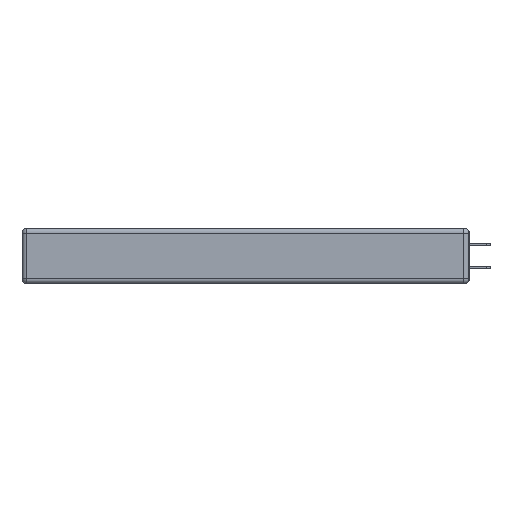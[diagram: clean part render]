
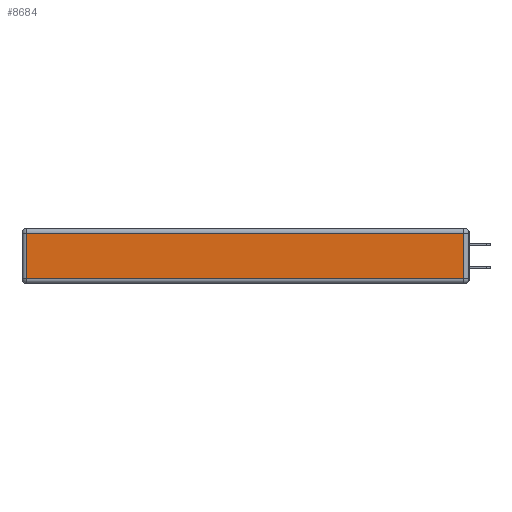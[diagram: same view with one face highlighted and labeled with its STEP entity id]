
A CAD part, left-side view. The second image highlights one B-rep face of the part: STEP entity #8684.
In plain terms, the highlighted planar face has unit normal (-1, 0, 0).
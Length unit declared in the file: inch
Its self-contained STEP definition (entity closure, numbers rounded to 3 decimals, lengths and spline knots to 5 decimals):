
#190 = LINE ( 'NONE', #18032, #3836 ) ;
#282 = DIRECTION ( 'NONE',  ( 0., 1., 0. ) ) ;
#2581 = VERTEX_POINT ( 'NONE', #12577 ) ;
#2840 = ORIENTED_EDGE ( 'NONE', *, *, #27368, .T. ) ;
#3521 = CARTESIAN_POINT ( 'NONE',  ( 0., 2.72, -0.313 ) ) ;
#3836 = VECTOR ( 'NONE', #12728, 39.37008 ) ;
#5255 = CARTESIAN_POINT ( 'NONE',  ( 0., 0.03, -0.313 ) ) ;
#5949 = VERTEX_POINT ( 'NONE', #33592 ) ;
#7208 = AXIS2_PLACEMENT_3D ( 'NONE', #22258, #24568, #11849 ) ;
#7485 = FACE_OUTER_BOUND ( 'NONE', #22815, .T. ) ;
#8135 = CARTESIAN_POINT ( 'NONE',  ( 0., 2.75, -0.03 ) ) ;
#8597 = CARTESIAN_POINT ( 'NONE',  ( 0., 2.72, -0.343 ) ) ;
#8684 = ADVANCED_FACE ( 'NONE', ( #7485 ), #8914, .T. ) ;
#8914 = PLANE ( 'NONE',  #7208 ) ;
#10251 = EDGE_CURVE ( 'NONE', #2581, #5949, #10608, .T. ) ;
#10278 = VECTOR ( 'NONE', #11177, 39.37008 ) ;
#10608 = LINE ( 'NONE', #8135, #11804 ) ;
#11177 = DIRECTION ( 'NONE',  ( 0., 0., -1. ) ) ;
#11804 = VECTOR ( 'NONE', #282, 39.37008 ) ;
#11849 = DIRECTION ( 'NONE',  ( 0., 0., 1. ) ) ;
#12577 = CARTESIAN_POINT ( 'NONE',  ( 0., 0.03, -0.03 ) ) ;
#12728 = DIRECTION ( 'NONE',  ( 0., -1., 0. ) ) ;
#15113 = ORIENTED_EDGE ( 'NONE', *, *, #27720, .T. ) ;
#15547 = VECTOR ( 'NONE', #23289, 39.37008 ) ;
#18032 = CARTESIAN_POINT ( 'NONE',  ( 0., 0., -0.313 ) ) ;
#20417 = VERTEX_POINT ( 'NONE', #5255 ) ;
#22258 = CARTESIAN_POINT ( 'NONE',  ( 0., 0., -0.343 ) ) ;
#22516 = LINE ( 'NONE', #23057, #15547 ) ;
#22815 = EDGE_LOOP ( 'NONE', ( #28916, #15113, #26119, #2840 ) ) ;
#23057 = CARTESIAN_POINT ( 'NONE',  ( 0., 0.03, -0.343 ) ) ;
#23289 = DIRECTION ( 'NONE',  ( 0., 0., 1. ) ) ;
#24568 = DIRECTION ( 'NONE',  ( -1., 0., 0. ) ) ;
#26119 = ORIENTED_EDGE ( 'NONE', *, *, #10251, .T. ) ;
#26668 = EDGE_CURVE ( 'NONE', #30975, #20417, #190, .T. ) ;
#27368 = EDGE_CURVE ( 'NONE', #5949, #30975, #33099, .T. ) ;
#27720 = EDGE_CURVE ( 'NONE', #20417, #2581, #22516, .T. ) ;
#28916 = ORIENTED_EDGE ( 'NONE', *, *, #26668, .T. ) ;
#30975 = VERTEX_POINT ( 'NONE', #3521 ) ;
#33099 = LINE ( 'NONE', #8597, #10278 ) ;
#33592 = CARTESIAN_POINT ( 'NONE',  ( 0., 2.72, -0.03 ) ) ;
